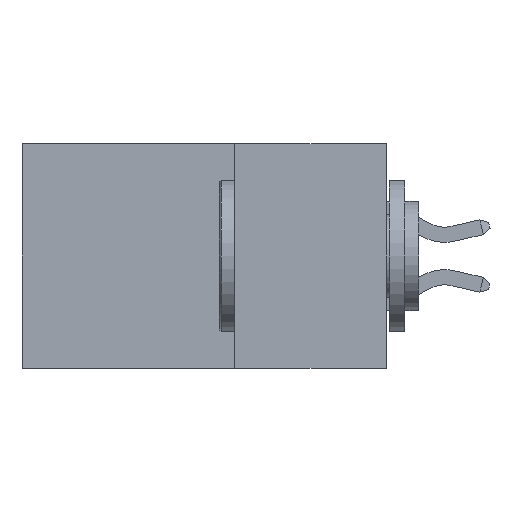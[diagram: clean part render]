
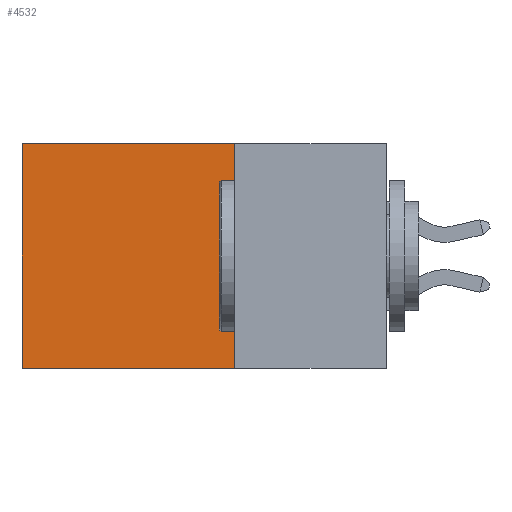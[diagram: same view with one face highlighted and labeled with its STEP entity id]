
A CAD part, left-side view. The second image highlights one B-rep face of the part: STEP entity #4532.
In plain terms, the highlighted planar face has unit normal (-1, 0, 0).
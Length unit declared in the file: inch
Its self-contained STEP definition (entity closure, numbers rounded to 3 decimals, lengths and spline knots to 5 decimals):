
#1488 = EDGE_CURVE ( 'NONE', #6578, #3568, #4751, .T. ) ;
#1615 = DIRECTION ( 'NONE',  ( 1., 0., 0. ) ) ;
#2179 = VERTEX_POINT ( 'NONE', #6848 ) ;
#2405 = ORIENTED_EDGE ( 'NONE', *, *, #10710, .F. ) ;
#3568 = VERTEX_POINT ( 'NONE', #4176 ) ;
#3814 = LINE ( 'NONE', #13318, #9413 ) ;
#3875 = FACE_OUTER_BOUND ( 'NONE', #12834, .T. ) ;
#4087 = DIRECTION ( 'NONE',  ( 0., 1., 0. ) ) ;
#4176 = CARTESIAN_POINT ( 'NONE',  ( 0.298, 0.6, 0. ) ) ;
#4532 = ADVANCED_FACE ( 'NONE', ( #3875 ), #5991, .F. ) ;
#4751 = LINE ( 'NONE', #5293, #7267 ) ;
#5183 = VECTOR ( 'NONE', #10903, 39.37008 ) ;
#5293 = CARTESIAN_POINT ( 'NONE',  ( 0.298, 0.25, 0. ) ) ;
#5455 = DIRECTION ( 'NONE',  ( 0., 0., -1. ) ) ;
#5792 = VECTOR ( 'NONE', #5455, 39.37008 ) ;
#5956 = CARTESIAN_POINT ( 'NONE',  ( 0.298, 0.25, 0. ) ) ;
#5991 = PLANE ( 'NONE',  #8779 ) ;
#6129 = LINE ( 'NONE', #9646, #5792 ) ;
#6364 = DIRECTION ( 'NONE',  ( 0., 0., -1. ) ) ;
#6578 = VERTEX_POINT ( 'NONE', #7910 ) ;
#6684 = ORIENTED_EDGE ( 'NONE', *, *, #1488, .T. ) ;
#6848 = CARTESIAN_POINT ( 'NONE',  ( 0.298, 0.6, -0.37 ) ) ;
#7149 = DIRECTION ( 'NONE',  ( 0., 0., -1. ) ) ;
#7267 = VECTOR ( 'NONE', #4087, 39.37008 ) ;
#7910 = CARTESIAN_POINT ( 'NONE',  ( 0.298, 0.25, 0. ) ) ;
#7963 = ORIENTED_EDGE ( 'NONE', *, *, #12403, .T. ) ;
#7987 = LINE ( 'NONE', #9861, #5183 ) ;
#7993 = VERTEX_POINT ( 'NONE', #11936 ) ;
#8779 = AXIS2_PLACEMENT_3D ( 'NONE', #5956, #1615, #6364 ) ;
#9413 = VECTOR ( 'NONE', #7149, 39.37008 ) ;
#9646 = CARTESIAN_POINT ( 'NONE',  ( 0.298, 0.6, 0. ) ) ;
#9861 = CARTESIAN_POINT ( 'NONE',  ( 0.298, 0.25, -0.37 ) ) ;
#10257 = ORIENTED_EDGE ( 'NONE', *, *, #12112, .F. ) ;
#10710 = EDGE_CURVE ( 'NONE', #7993, #2179, #7987, .T. ) ;
#10903 = DIRECTION ( 'NONE',  ( 0., 1., 0. ) ) ;
#11936 = CARTESIAN_POINT ( 'NONE',  ( 0.298, 0.25, -0.37 ) ) ;
#12112 = EDGE_CURVE ( 'NONE', #6578, #7993, #3814, .T. ) ;
#12403 = EDGE_CURVE ( 'NONE', #3568, #2179, #6129, .T. ) ;
#12834 = EDGE_LOOP ( 'NONE', ( #7963, #2405, #10257, #6684 ) ) ;
#13318 = CARTESIAN_POINT ( 'NONE',  ( 0.298, 0.25, 0. ) ) ;
